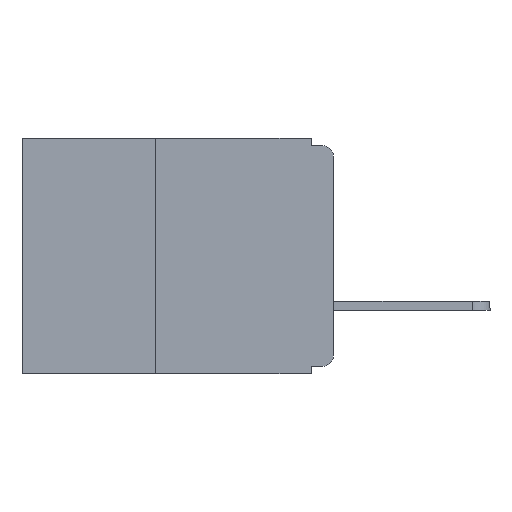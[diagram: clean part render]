
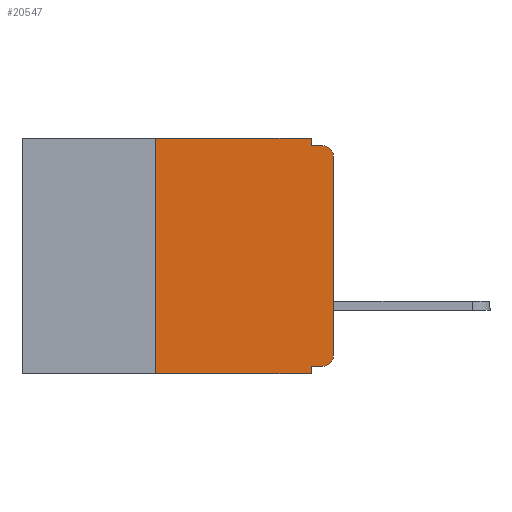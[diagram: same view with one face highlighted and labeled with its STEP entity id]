
A CAD part, left-side view. The second image highlights one B-rep face of the part: STEP entity #20547.
In plain terms, the highlighted planar face has unit normal (-1, 0, 0).
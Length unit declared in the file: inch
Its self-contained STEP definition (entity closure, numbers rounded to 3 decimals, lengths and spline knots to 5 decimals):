
#1055 = EDGE_CURVE ( 'NONE', #5716, #29247, #20704, .T. ) ;
#1470 = LINE ( 'NONE', #7629, #18935 ) ;
#1493 = ORIENTED_EDGE ( 'NONE', *, *, #5090, .T. ) ;
#1654 = VERTEX_POINT ( 'NONE', #1764 ) ;
#1742 = VECTOR ( 'NONE', #10643, 39.37008 ) ;
#1764 = CARTESIAN_POINT ( 'NONE',  ( 0., 0.015, -0.32 ) ) ;
#1881 = EDGE_CURVE ( 'NONE', #25248, #16716, #15012, .T. ) ;
#2533 = DIRECTION ( 'NONE',  ( 0., 0., -1. ) ) ;
#2569 = DIRECTION ( 'NONE',  ( -1., 0., 0. ) ) ;
#2572 = CARTESIAN_POINT ( 'NONE',  ( 0., 0.015, -0.025 ) ) ;
#2793 = DIRECTION ( 'NONE',  ( 0., 0., 1. ) ) ;
#4011 = DIRECTION ( 'NONE',  ( 0., 0., 1. ) ) ;
#4312 = LINE ( 'NONE', #8376, #16197 ) ;
#4849 = CARTESIAN_POINT ( 'NONE',  ( 0., 0., 0. ) ) ;
#5090 = EDGE_CURVE ( 'NONE', #28088, #23639, #25820, .T. ) ;
#5586 = VERTEX_POINT ( 'NONE', #26914 ) ;
#5716 = VERTEX_POINT ( 'NONE', #6688 ) ;
#5957 = EDGE_CURVE ( 'NONE', #16716, #29247, #7536, .T. ) ;
#6688 = CARTESIAN_POINT ( 'NONE',  ( 0., 0.031, -0.01 ) ) ;
#7291 = AXIS2_PLACEMENT_3D ( 'NONE', #26672, #12471, #29036 ) ;
#7395 = CARTESIAN_POINT ( 'NONE',  ( 0., 0.015, -0.305 ) ) ;
#7445 = EDGE_CURVE ( 'NONE', #1654, #5586, #8515, .T. ) ;
#7536 = CIRCLE ( 'NONE', #25437, 0.015 ) ;
#7629 = CARTESIAN_POINT ( 'NONE',  ( 0., 0.031, 0. ) ) ;
#7731 = ORIENTED_EDGE ( 'NONE', *, *, #25085, .F. ) ;
#7749 = DIRECTION ( 'NONE',  ( 0., -1., 0. ) ) ;
#7921 = CARTESIAN_POINT ( 'NONE',  ( 0., 0.437, 0. ) ) ;
#8032 = EDGE_CURVE ( 'NONE', #17836, #19561, #14425, .T. ) ;
#8376 = CARTESIAN_POINT ( 'NONE',  ( 0., 0.031, -0.33 ) ) ;
#8515 = LINE ( 'NONE', #20407, #26713 ) ;
#8690 = VECTOR ( 'NONE', #4011, 39.37008 ) ;
#8747 = DIRECTION ( 'NONE',  ( 0., -1., 0. ) ) ;
#9736 = DIRECTION ( 'NONE',  ( 0., 0., -1. ) ) ;
#9821 = CARTESIAN_POINT ( 'NONE',  ( 0., 0.25, -0.33 ) ) ;
#9857 = CARTESIAN_POINT ( 'NONE',  ( 0., 0.437, -0.33 ) ) ;
#9966 = FACE_OUTER_BOUND ( 'NONE', #12459, .T. ) ;
#9975 = DIRECTION ( 'NONE',  ( 0., 0., -1. ) ) ;
#10643 = DIRECTION ( 'NONE',  ( 0., -1., 0. ) ) ;
#10768 = DIRECTION ( 'NONE',  ( 0., 0., -1. ) ) ;
#11481 = ORIENTED_EDGE ( 'NONE', *, *, #7445, .F. ) ;
#11848 = ORIENTED_EDGE ( 'NONE', *, *, #19384, .F. ) ;
#11916 = LINE ( 'NONE', #9821, #23827 ) ;
#12459 = EDGE_LOOP ( 'NONE', ( #12970, #17507, #12537, #7731, #20058, #11848, #1493, #21206, #11481, #21603 ) ) ;
#12471 = DIRECTION ( 'NONE',  ( 1., 0., 0. ) ) ;
#12537 = ORIENTED_EDGE ( 'NONE', *, *, #1055, .F. ) ;
#12970 = ORIENTED_EDGE ( 'NONE', *, *, #1881, .T. ) ;
#13735 = CARTESIAN_POINT ( 'NONE',  ( 0., 0.031, -0.33 ) ) ;
#14213 = EDGE_CURVE ( 'NONE', #5586, #23639, #4312, .T. ) ;
#14425 = LINE ( 'NONE', #7921, #20804 ) ;
#15012 = LINE ( 'NONE', #4849, #8690 ) ;
#16197 = VECTOR ( 'NONE', #10768, 39.37008 ) ;
#16716 = VERTEX_POINT ( 'NONE', #23812 ) ;
#17261 = CIRCLE ( 'NONE', #28405, 0.015 ) ;
#17507 = ORIENTED_EDGE ( 'NONE', *, *, #5957, .T. ) ;
#17836 = VERTEX_POINT ( 'NONE', #30118 ) ;
#17909 = CARTESIAN_POINT ( 'NONE',  ( 0., 0.25, -0.33 ) ) ;
#18935 = VECTOR ( 'NONE', #9975, 39.37008 ) ;
#19384 = EDGE_CURVE ( 'NONE', #28088, #17836, #11916, .T. ) ;
#19561 = VERTEX_POINT ( 'NONE', #20572 ) ;
#20058 = ORIENTED_EDGE ( 'NONE', *, *, #8032, .F. ) ;
#20268 = DIRECTION ( 'NONE',  ( 0., 1., 0. ) ) ;
#20407 = CARTESIAN_POINT ( 'NONE',  ( 0., 0., -0.32 ) ) ;
#20547 = ADVANCED_FACE ( 'NONE', ( #9966 ), #28928, .F. ) ;
#20572 = CARTESIAN_POINT ( 'NONE',  ( 0., 0.031, 0. ) ) ;
#20704 = LINE ( 'NONE', #21201, #1742 ) ;
#20804 = VECTOR ( 'NONE', #7749, 39.37008 ) ;
#21201 = CARTESIAN_POINT ( 'NONE',  ( 0., 0., -0.01 ) ) ;
#21206 = ORIENTED_EDGE ( 'NONE', *, *, #14213, .F. ) ;
#21603 = ORIENTED_EDGE ( 'NONE', *, *, #28431, .T. ) ;
#23639 = VERTEX_POINT ( 'NONE', #13735 ) ;
#23812 = CARTESIAN_POINT ( 'NONE',  ( 0., 0., -0.025 ) ) ;
#23827 = VECTOR ( 'NONE', #2793, 39.37008 ) ;
#23989 = DIRECTION ( 'NONE',  ( -1., 0., 0. ) ) ;
#25073 = VECTOR ( 'NONE', #8747, 39.37008 ) ;
#25085 = EDGE_CURVE ( 'NONE', #19561, #5716, #1470, .T. ) ;
#25248 = VERTEX_POINT ( 'NONE', #29459 ) ;
#25437 = AXIS2_PLACEMENT_3D ( 'NONE', #2572, #2569, #2533 ) ;
#25820 = LINE ( 'NONE', #9857, #25073 ) ;
#26672 = CARTESIAN_POINT ( 'NONE',  ( 0., 0.437, 0. ) ) ;
#26713 = VECTOR ( 'NONE', #20268, 39.37008 ) ;
#26914 = CARTESIAN_POINT ( 'NONE',  ( 0., 0.031, -0.32 ) ) ;
#27860 = CARTESIAN_POINT ( 'NONE',  ( 0., 0.015, -0.01 ) ) ;
#28088 = VERTEX_POINT ( 'NONE', #17909 ) ;
#28405 = AXIS2_PLACEMENT_3D ( 'NONE', #7395, #23989, #9736 ) ;
#28431 = EDGE_CURVE ( 'NONE', #1654, #25248, #17261, .T. ) ;
#28928 = PLANE ( 'NONE',  #7291 ) ;
#29036 = DIRECTION ( 'NONE',  ( 0., 0., -1. ) ) ;
#29247 = VERTEX_POINT ( 'NONE', #27860 ) ;
#29459 = CARTESIAN_POINT ( 'NONE',  ( 0., 0., -0.305 ) ) ;
#30118 = CARTESIAN_POINT ( 'NONE',  ( 0., 0.25, 0. ) ) ;
